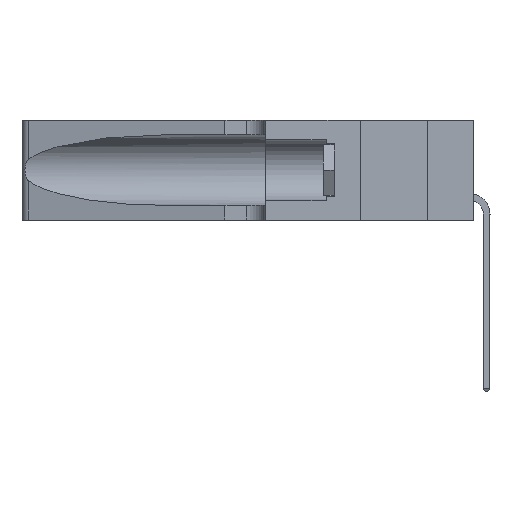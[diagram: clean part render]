
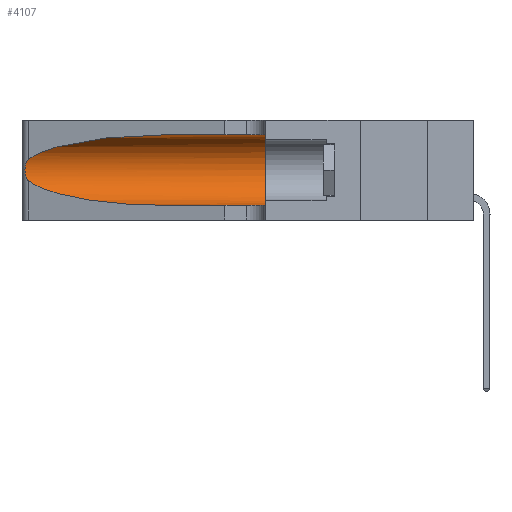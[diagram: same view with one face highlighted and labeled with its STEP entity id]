
A CAD part, left-side view. The second image highlights one B-rep face of the part: STEP entity #4107.
In plain terms, the highlighted cylindrical face has radius 3.308 mm (diameter 6.617 mm), a partial arc.
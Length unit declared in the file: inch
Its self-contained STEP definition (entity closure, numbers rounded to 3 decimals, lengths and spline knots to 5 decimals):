
#34 = CARTESIAN_POINT ( 'NONE',  ( 0.1305, 1.61858, 0.05475 ) ) ;
#250 = ORIENTED_EDGE ( 'NONE', *, *, #1273, .T. ) ;
#392 = EDGE_CURVE ( 'NONE', #2080, #1799, #6456, .T. ) ;
#698 = CARTESIAN_POINT ( 'NONE',  ( 0.25487, 1.22718, 0.14631 ) ) ;
#773 = VERTEX_POINT ( 'NONE', #698 ) ;
#1273 = EDGE_CURVE ( 'NONE', #16684, #13300, #17404, .T. ) ;
#1407 = CARTESIAN_POINT ( 'NONE',  ( 0.25555, 1.22994, 0.2215 ) ) ;
#1793 = CARTESIAN_POINT ( 'NONE',  ( 0.1305, 1.61858, 0.185 ) ) ;
#1799 = VERTEX_POINT ( 'NONE', #7361 ) ;
#2080 = VERTEX_POINT ( 'NONE', #2522 ) ;
#2410 = EDGE_CURVE ( 'NONE', #773, #16684, #9894, .T. ) ;
#2522 = CARTESIAN_POINT ( 'NONE',  ( 0.1305, 0.72297, 0.31525 ) ) ;
#2608 = CARTESIAN_POINT ( 'NONE',  ( 0.25639, 1.23184, 0.21858 ) ) ;
#2660 = CARTESIAN_POINT ( 'NONE',  ( 0.26075, 1.23896, 0.19203 ) ) ;
#3117 = ORIENTED_EDGE ( 'NONE', *, *, #2410, .T. ) ;
#3159 = DIRECTION ( 'NONE',  ( 0., -1., 0. ) ) ;
#3652 = LINE ( 'NONE', #16101, #14709 ) ;
#3990 = CARTESIAN_POINT ( 'NONE',  ( 0.25555, 1.22993, 0.14849 ) ) ;
#4107 = ADVANCED_FACE ( 'NONE', ( #9195 ), #7003, .F. ) ;
#4135 = CIRCLE ( 'NONE', #16905, 0.13025 ) ;
#4251 = DIRECTION ( 'NONE',  ( 0., -1., 0. ) ) ;
#4967 = CARTESIAN_POINT ( 'NONE',  ( 0.1305, 0.72297, 0.05475 ) ) ;
#5594 = DIRECTION ( 'NONE',  ( 0., 1., 0. ) ) ;
#5788 = EDGE_CURVE ( 'NONE', #1799, #773, #15215, .T. ) ;
#6256 = CARTESIAN_POINT ( 'NONE',  ( 0.1305, 0.72297, 0.05475 ) ) ;
#6293 = CARTESIAN_POINT ( 'NONE',  ( 0.1305, 0.35, 0.05475 ) ) ;
#6456 =( BOUNDED_CURVE ( )  B_SPLINE_CURVE ( 3, ( #10620, #11979, #6519, #17513 ),
 .UNSPECIFIED., .F., .F. ) 
 B_SPLINE_CURVE_WITH_KNOTS ( ( 4, 4 ),
 ( 1.5708, 2.84003 ),
 .UNSPECIFIED. ) 
 CURVE ( )  GEOMETRIC_REPRESENTATION_ITEM ( )  RATIONAL_B_SPLINE_CURVE ( ( 1., 0.87, 0.87, 1. ) ) 
 REPRESENTATION_ITEM ( '' )  );
#6519 = CARTESIAN_POINT ( 'NONE',  ( 0.2373, 1.15595, 0.28018 ) ) ;
#6732 = CARTESIAN_POINT ( 'NONE',  ( 0.25856, 1.23593, 0.16098 ) ) ;
#6958 = CARTESIAN_POINT ( 'NONE',  ( 0.25854, 1.2359, 0.20912 ) ) ;
#7003 = CYLINDRICAL_SURFACE ( 'NONE', #16846, 0.13025 ) ;
#7257 = VECTOR ( 'NONE', #4251, 39.37008 ) ;
#7361 = CARTESIAN_POINT ( 'NONE',  ( 0.25487, 1.22718, 0.22369 ) ) ;
#7455 = EDGE_CURVE ( 'NONE', #2080, #12376, #3652, .T. ) ;
#7581 = CARTESIAN_POINT ( 'NONE',  ( 0.18966, 0.96281, 0.05475 ) ) ;
#7832 = EDGE_LOOP ( 'NONE', ( #14436, #9339, #3117, #250, #14676, #10641 ) ) ;
#8215 = CARTESIAN_POINT ( 'NONE',  ( 0.26017, 1.23833, 0.17102 ) ) ;
#9145 = EDGE_CURVE ( 'NONE', #12376, #13300, #4135, .T. ) ;
#9195 = FACE_OUTER_BOUND ( 'NONE', #7832, .T. ) ;
#9339 = ORIENTED_EDGE ( 'NONE', *, *, #5788, .T. ) ;
#9568 = CARTESIAN_POINT ( 'NONE',  ( 0.25487, 1.22718, 0.22369 ) ) ;
#9879 = DIRECTION ( 'NONE',  ( 0., 0., 1. ) ) ;
#9894 =( BOUNDED_CURVE ( )  B_SPLINE_CURVE ( 3, ( #11654, #10129, #7581, #6256 ),
 .UNSPECIFIED., .F., .T. ) 
 B_SPLINE_CURVE_WITH_KNOTS ( ( 4, 4 ),
 ( 3.44316, 4.71239 ),
 .UNSPECIFIED. ) 
 CURVE ( )  GEOMETRIC_REPRESENTATION_ITEM ( )  RATIONAL_B_SPLINE_CURVE ( ( 1., 0.87, 0.87, 1. ) ) 
 REPRESENTATION_ITEM ( '' )  );
#10129 = CARTESIAN_POINT ( 'NONE',  ( 0.2373, 1.15595, 0.08982 ) ) ;
#10620 = CARTESIAN_POINT ( 'NONE',  ( 0.1305, 0.72297, 0.31525 ) ) ;
#10641 = ORIENTED_EDGE ( 'NONE', *, *, #7455, .F. ) ;
#10889 = CARTESIAN_POINT ( 'NONE',  ( 0.1305, 0.35, 0.31525 ) ) ;
#10899 = CARTESIAN_POINT ( 'NONE',  ( 0.25639, 1.23186, 0.15144 ) ) ;
#10961 = CARTESIAN_POINT ( 'NONE',  ( 0.25787, 1.23484, 0.2124 ) ) ;
#11654 = CARTESIAN_POINT ( 'NONE',  ( 0.25487, 1.22718, 0.14631 ) ) ;
#11979 = CARTESIAN_POINT ( 'NONE',  ( 0.18966, 0.96281, 0.31525 ) ) ;
#12305 = CARTESIAN_POINT ( 'NONE',  ( 0.26018, 1.23835, 0.19895 ) ) ;
#12376 = VERTEX_POINT ( 'NONE', #10889 ) ;
#12537 = CARTESIAN_POINT ( 'NONE',  ( 0.25487, 1.22718, 0.14631 ) ) ;
#12871 = DIRECTION ( 'NONE',  ( 0., 0., -1. ) ) ;
#13295 = DIRECTION ( 'NONE',  ( 0., -1., 0. ) ) ;
#13300 = VERTEX_POINT ( 'NONE', #6293 ) ;
#14436 = ORIENTED_EDGE ( 'NONE', *, *, #392, .T. ) ;
#14676 = ORIENTED_EDGE ( 'NONE', *, *, #9145, .F. ) ;
#14709 = VECTOR ( 'NONE', #13295, 39.37008 ) ;
#15188 = CARTESIAN_POINT ( 'NONE',  ( 0.26075, 1.23896, 0.178 ) ) ;
#15215 = B_SPLINE_CURVE_WITH_KNOTS ( 'NONE', 3,
 ( #9568, #1407, #2608, #10961, #6958, #12305, #2660, #15188, #8215, #6732, #17923, #10899, #3990, #12537 ),
 .UNSPECIFIED., .F., .F.,
 ( 4, 2, 2, 2, 2, 2, 4 ),
 ( 0., 0.00027, 0.00053, 0.00107, 0.0016, 0.00187, 0.00214 ),
 .UNSPECIFIED. ) ;
#15385 = CARTESIAN_POINT ( 'NONE',  ( 0.1305, 0.35, 0.185 ) ) ;
#16101 = CARTESIAN_POINT ( 'NONE',  ( 0.1305, 1.61858, 0.31525 ) ) ;
#16684 = VERTEX_POINT ( 'NONE', #4967 ) ;
#16846 = AXIS2_PLACEMENT_3D ( 'NONE', #1793, #3159, #12871 ) ;
#16905 = AXIS2_PLACEMENT_3D ( 'NONE', #15385, #5594, #9879 ) ;
#17404 = LINE ( 'NONE', #34, #7257 ) ;
#17513 = CARTESIAN_POINT ( 'NONE',  ( 0.25487, 1.22718, 0.22369 ) ) ;
#17923 = CARTESIAN_POINT ( 'NONE',  ( 0.25789, 1.23486, 0.15765 ) ) ;
